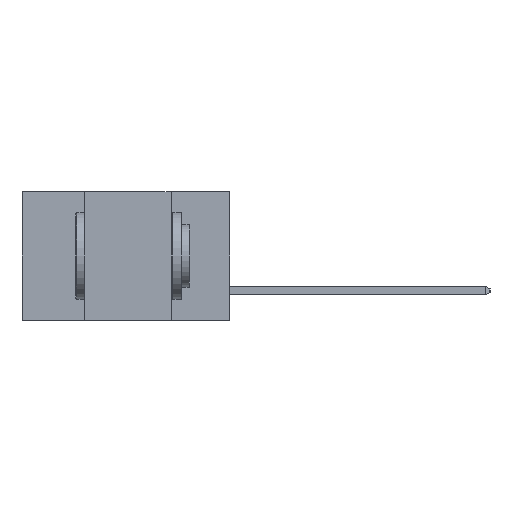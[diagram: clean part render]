
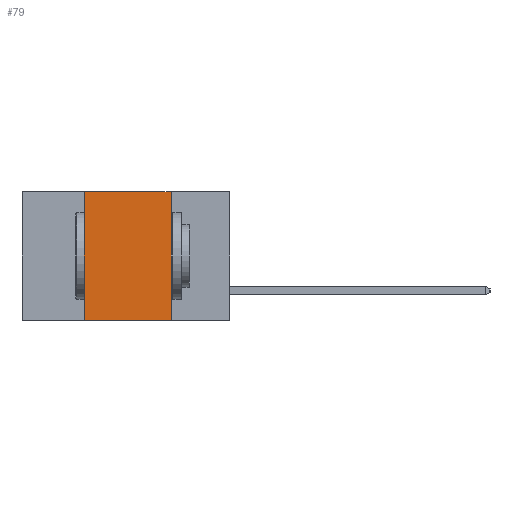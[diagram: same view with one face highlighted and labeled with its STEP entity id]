
A CAD part, left-side view. The second image highlights one B-rep face of the part: STEP entity #79.
In plain terms, the highlighted planar face has unit normal (-1, 0, 0).
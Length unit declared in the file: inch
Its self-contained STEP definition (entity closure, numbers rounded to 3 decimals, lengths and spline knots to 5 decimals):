
#79 = ADVANCED_FACE ( 'NONE', ( #11122 ), #18821, .F. ) ;
#1338 = DIRECTION ( 'NONE',  ( 0., -1., 0. ) ) ;
#1580 = ORIENTED_EDGE ( 'NONE', *, *, #10660, .T. ) ;
#1639 = DIRECTION ( 'NONE',  ( 0., -1., 0. ) ) ;
#1731 = CARTESIAN_POINT ( 'NONE',  ( 0., 0.6, 0. ) ) ;
#2164 = VECTOR ( 'NONE', #1338, 39.37008 ) ;
#2388 = LINE ( 'NONE', #5215, #9603 ) ;
#2466 = EDGE_LOOP ( 'NONE', ( #5873, #10501, #12912, #1580 ) ) ;
#2809 = VERTEX_POINT ( 'NONE', #18506 ) ;
#3050 = CARTESIAN_POINT ( 'NONE',  ( 0., 0.6, -0.37 ) ) ;
#3964 = CARTESIAN_POINT ( 'NONE',  ( 0., 0.17, 0. ) ) ;
#5215 = CARTESIAN_POINT ( 'NONE',  ( 0., 0.42, 0. ) ) ;
#5240 = DIRECTION ( 'NONE',  ( 0., 0., 1. ) ) ;
#5318 = EDGE_CURVE ( 'NONE', #16010, #2809, #17492, .T. ) ;
#5551 = EDGE_CURVE ( 'NONE', #11022, #16010, #2388, .T. ) ;
#5873 = ORIENTED_EDGE ( 'NONE', *, *, #11701, .F. ) ;
#8465 = AXIS2_PLACEMENT_3D ( 'NONE', #13476, #14816, #14781 ) ;
#8563 = DIRECTION ( 'NONE',  ( 0., 0., -1. ) ) ;
#9603 = VECTOR ( 'NONE', #5240, 39.37008 ) ;
#10501 = ORIENTED_EDGE ( 'NONE', *, *, #5318, .F. ) ;
#10660 = EDGE_CURVE ( 'NONE', #11022, #14518, #14809, .T. ) ;
#11022 = VERTEX_POINT ( 'NONE', #17770 ) ;
#11122 = FACE_OUTER_BOUND ( 'NONE', #2466, .T. ) ;
#11415 = VECTOR ( 'NONE', #8563, 39.37008 ) ;
#11701 = EDGE_CURVE ( 'NONE', #2809, #14518, #19438, .T. ) ;
#11972 = CARTESIAN_POINT ( 'NONE',  ( 0., 0.42, 0. ) ) ;
#12912 = ORIENTED_EDGE ( 'NONE', *, *, #5551, .F. ) ;
#13476 = CARTESIAN_POINT ( 'NONE',  ( 0., 0.6, 0. ) ) ;
#14242 = CARTESIAN_POINT ( 'NONE',  ( 0., 0.17, -0.37 ) ) ;
#14338 = VECTOR ( 'NONE', #1639, 39.37008 ) ;
#14518 = VERTEX_POINT ( 'NONE', #14242 ) ;
#14781 = DIRECTION ( 'NONE',  ( 0., 0., -1. ) ) ;
#14809 = LINE ( 'NONE', #3050, #14338 ) ;
#14816 = DIRECTION ( 'NONE',  ( 1., 0., 0. ) ) ;
#16010 = VERTEX_POINT ( 'NONE', #11972 ) ;
#17492 = LINE ( 'NONE', #1731, #2164 ) ;
#17770 = CARTESIAN_POINT ( 'NONE',  ( 0., 0.42, -0.37 ) ) ;
#18506 = CARTESIAN_POINT ( 'NONE',  ( 0., 0.17, 0. ) ) ;
#18821 = PLANE ( 'NONE',  #8465 ) ;
#19438 = LINE ( 'NONE', #3964, #11415 ) ;
